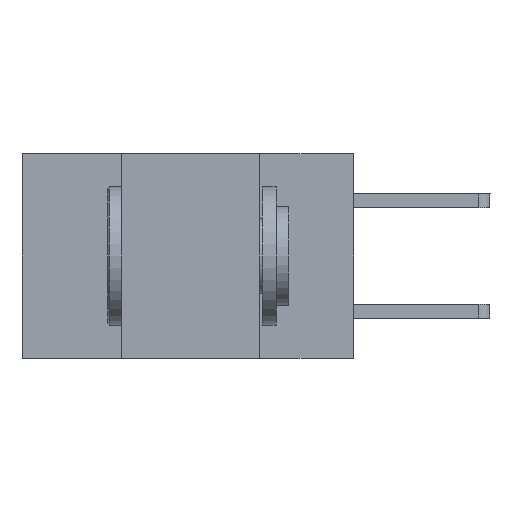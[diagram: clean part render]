
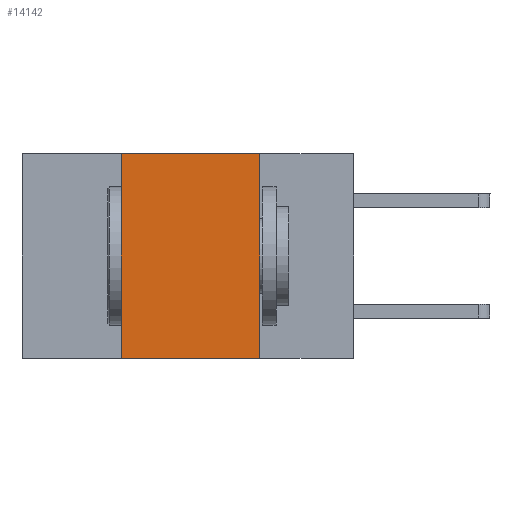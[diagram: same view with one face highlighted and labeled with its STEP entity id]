
A CAD part, left-side view. The second image highlights one B-rep face of the part: STEP entity #14142.
In plain terms, the highlighted planar face has unit normal (-1, 0, 0).
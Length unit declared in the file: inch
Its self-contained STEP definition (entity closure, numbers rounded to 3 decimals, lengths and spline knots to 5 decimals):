
#270 = LINE ( 'NONE', #6413, #9184 ) ;
#973 = DIRECTION ( 'NONE',  ( 0., 0., 1. ) ) ;
#1106 = CARTESIAN_POINT ( 'NONE',  ( 0., 0.17, -0.37 ) ) ;
#1581 = PLANE ( 'NONE',  #12031 ) ;
#1606 = CARTESIAN_POINT ( 'NONE',  ( 0., 0.42, 0. ) ) ;
#2336 = CARTESIAN_POINT ( 'NONE',  ( 0., 0.6, 0. ) ) ;
#3563 = DIRECTION ( 'NONE',  ( 0., 0., -1. ) ) ;
#3768 = CARTESIAN_POINT ( 'NONE',  ( 0., 0.6, 0. ) ) ;
#4152 = DIRECTION ( 'NONE',  ( 0., -1., 0. ) ) ;
#4478 = DIRECTION ( 'NONE',  ( 0., -1., 0. ) ) ;
#5241 = ORIENTED_EDGE ( 'NONE', *, *, #8580, .F. ) ;
#5884 = DIRECTION ( 'NONE',  ( 0., 0., -1. ) ) ;
#6122 = FACE_OUTER_BOUND ( 'NONE', #10239, .T. ) ;
#6213 = LINE ( 'NONE', #2336, #7062 ) ;
#6413 = CARTESIAN_POINT ( 'NONE',  ( 0., 0.42, 0. ) ) ;
#6802 = VERTEX_POINT ( 'NONE', #1606 ) ;
#7062 = VECTOR ( 'NONE', #4478, 39.37008 ) ;
#7420 = CARTESIAN_POINT ( 'NONE',  ( 0., 0.6, -0.37 ) ) ;
#7837 = VERTEX_POINT ( 'NONE', #11793 ) ;
#7921 = EDGE_CURVE ( 'NONE', #9009, #12080, #7995, .T. ) ;
#7995 = LINE ( 'NONE', #7420, #13479 ) ;
#8580 = EDGE_CURVE ( 'NONE', #9009, #6802, #270, .T. ) ;
#9009 = VERTEX_POINT ( 'NONE', #12587 ) ;
#9184 = VECTOR ( 'NONE', #973, 39.37008 ) ;
#9296 = ORIENTED_EDGE ( 'NONE', *, *, #7921, .T. ) ;
#9726 = EDGE_CURVE ( 'NONE', #7837, #12080, #12188, .T. ) ;
#9934 = VECTOR ( 'NONE', #3563, 39.37008 ) ;
#10079 = CARTESIAN_POINT ( 'NONE',  ( 0., 0.17, 0. ) ) ;
#10223 = DIRECTION ( 'NONE',  ( 1., 0., 0. ) ) ;
#10239 = EDGE_LOOP ( 'NONE', ( #12129, #10535, #5241, #9296 ) ) ;
#10353 = EDGE_CURVE ( 'NONE', #6802, #7837, #6213, .T. ) ;
#10535 = ORIENTED_EDGE ( 'NONE', *, *, #10353, .F. ) ;
#11793 = CARTESIAN_POINT ( 'NONE',  ( 0., 0.17, 0. ) ) ;
#12031 = AXIS2_PLACEMENT_3D ( 'NONE', #3768, #10223, #5884 ) ;
#12080 = VERTEX_POINT ( 'NONE', #1106 ) ;
#12129 = ORIENTED_EDGE ( 'NONE', *, *, #9726, .F. ) ;
#12188 = LINE ( 'NONE', #10079, #9934 ) ;
#12587 = CARTESIAN_POINT ( 'NONE',  ( 0., 0.42, -0.37 ) ) ;
#13479 = VECTOR ( 'NONE', #4152, 39.37008 ) ;
#14142 = ADVANCED_FACE ( 'NONE', ( #6122 ), #1581, .F. ) ;
